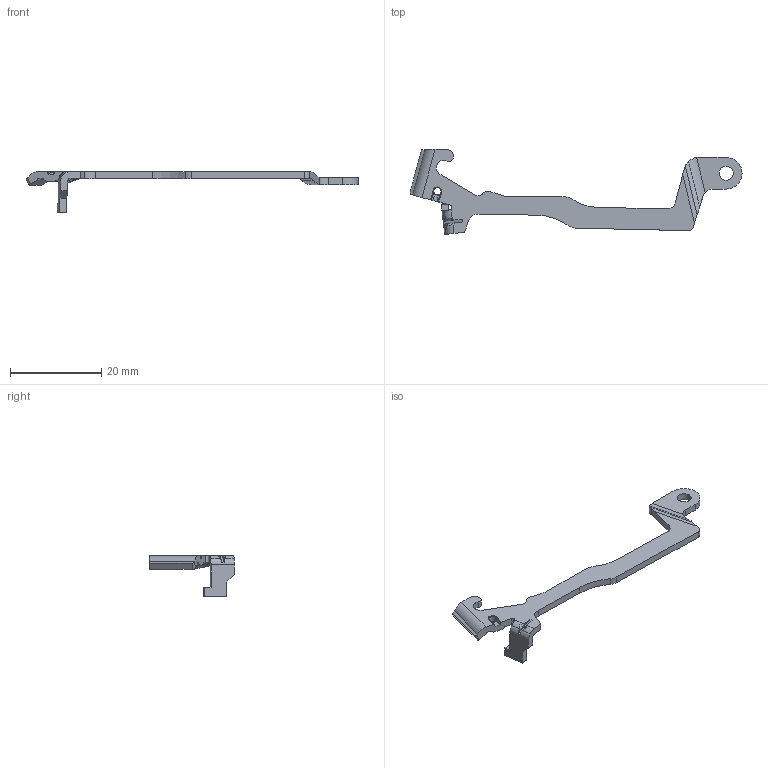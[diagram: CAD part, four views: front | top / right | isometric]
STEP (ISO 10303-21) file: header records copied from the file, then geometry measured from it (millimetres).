
FILE_DESCRIPTION (( 'STEP AP214' ), '1' );
FILE_NAME ('Trigger Bar.step', '2014-07-30T19:47:08', ( 'WarFairy' ), ( '' ), 'SwSTEP 2.0', 'SolidWorks 2013', '' );
FILE_SCHEMA (( 'AUTOMOTIVE_DESIGN' ));
Length unit declared in the file: millimetre
Products named in the file (1): Trigger Bar
Bounding box: 72.81 x 18.63 x 8.93 mm (x, y, z)
Volume: 763.8 mm3; surface area: 1346 mm2
Topology: 1 solids, 1 shells, 112 faces, 324 edges, 212 vertices
Faces by surface type: cylinder 58, plane 44, bspline 7, torus 3
Entity records: 4097 total; most frequent: CARTESIAN_POINT 1189, ORIENTED_EDGE 648, DIRECTION 560, EDGE_CURVE 324, VERTEX_POINT 212, AXIS2_PLACEMENT_3D 193, VECTOR 174, LINE 174
